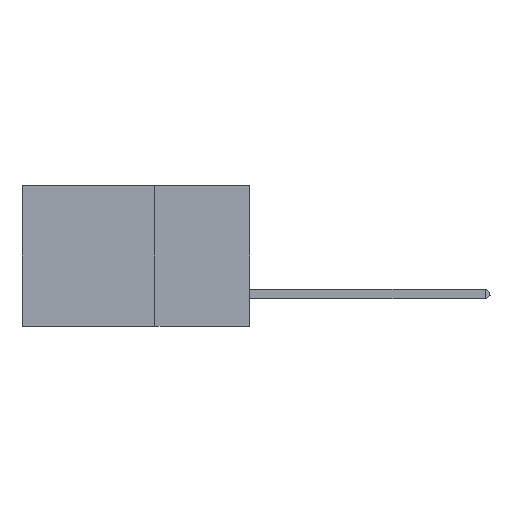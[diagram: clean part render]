
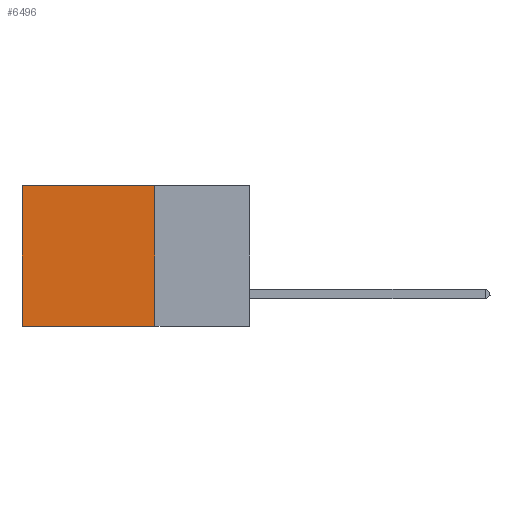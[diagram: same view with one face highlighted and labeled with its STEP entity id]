
A CAD part, left-side view. The second image highlights one B-rep face of the part: STEP entity #6496.
In plain terms, the highlighted planar face has unit normal (-1, 0, 0).
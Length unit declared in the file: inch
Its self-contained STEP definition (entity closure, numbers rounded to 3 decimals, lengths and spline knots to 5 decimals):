
#478 = CARTESIAN_POINT ( 'NONE',  ( 0.2875, 0.6, 0. ) ) ;
#818 = LINE ( 'NONE', #19215, #13894 ) ;
#987 = ORIENTED_EDGE ( 'NONE', *, *, #17618, .F. ) ;
#1534 = DIRECTION ( 'NONE',  ( 0., 0., -1. ) ) ;
#2122 = CARTESIAN_POINT ( 'NONE',  ( 0.2875, 0.6, -0.37 ) ) ;
#3192 = CARTESIAN_POINT ( 'NONE',  ( 0.2875, 0.6, 0. ) ) ;
#4718 = CARTESIAN_POINT ( 'NONE',  ( 0.2875, 0.25, 0. ) ) ;
#6496 = ADVANCED_FACE ( 'NONE', ( #13296 ), #9702, .F. ) ;
#7310 = DIRECTION ( 'NONE',  ( 0., 1., 0. ) ) ;
#8694 = EDGE_CURVE ( 'NONE', #19123, #15430, #818, .T. ) ;
#8834 = VERTEX_POINT ( 'NONE', #17411 ) ;
#9702 = PLANE ( 'NONE',  #15136 ) ;
#9778 = DIRECTION ( 'NONE',  ( 0., 1., 0. ) ) ;
#10836 = DIRECTION ( 'NONE',  ( 0., 0., -1. ) ) ;
#11532 = EDGE_CURVE ( 'NONE', #15180, #15430, #16863, .T. ) ;
#12886 = LINE ( 'NONE', #16772, #18801 ) ;
#13113 = EDGE_LOOP ( 'NONE', ( #15323, #18420, #987, #16323 ) ) ;
#13296 = FACE_OUTER_BOUND ( 'NONE', #13113, .T. ) ;
#13864 = VECTOR ( 'NONE', #15732, 39.37008 ) ;
#13894 = VECTOR ( 'NONE', #9778, 39.37008 ) ;
#15136 = AXIS2_PLACEMENT_3D ( 'NONE', #4718, #17409, #1534 ) ;
#15180 = VERTEX_POINT ( 'NONE', #478 ) ;
#15323 = ORIENTED_EDGE ( 'NONE', *, *, #11532, .T. ) ;
#15430 = VERTEX_POINT ( 'NONE', #2122 ) ;
#15732 = DIRECTION ( 'NONE',  ( 0., 0., -1. ) ) ;
#16323 = ORIENTED_EDGE ( 'NONE', *, *, #18126, .T. ) ;
#16772 = CARTESIAN_POINT ( 'NONE',  ( 0.2875, 0.25, 0. ) ) ;
#16863 = LINE ( 'NONE', #3192, #13864 ) ;
#17323 = CARTESIAN_POINT ( 'NONE',  ( 0.2875, 0.25, 0. ) ) ;
#17409 = DIRECTION ( 'NONE',  ( 1., 0., 0. ) ) ;
#17411 = CARTESIAN_POINT ( 'NONE',  ( 0.2875, 0.25, 0. ) ) ;
#17514 = CARTESIAN_POINT ( 'NONE',  ( 0.2875, 0.25, -0.37 ) ) ;
#17618 = EDGE_CURVE ( 'NONE', #8834, #19123, #18342, .T. ) ;
#18126 = EDGE_CURVE ( 'NONE', #8834, #15180, #12886, .T. ) ;
#18342 = LINE ( 'NONE', #17323, #18833 ) ;
#18420 = ORIENTED_EDGE ( 'NONE', *, *, #8694, .F. ) ;
#18801 = VECTOR ( 'NONE', #7310, 39.37008 ) ;
#18833 = VECTOR ( 'NONE', #10836, 39.37008 ) ;
#19123 = VERTEX_POINT ( 'NONE', #17514 ) ;
#19215 = CARTESIAN_POINT ( 'NONE',  ( 0.2875, 0.25, -0.37 ) ) ;
